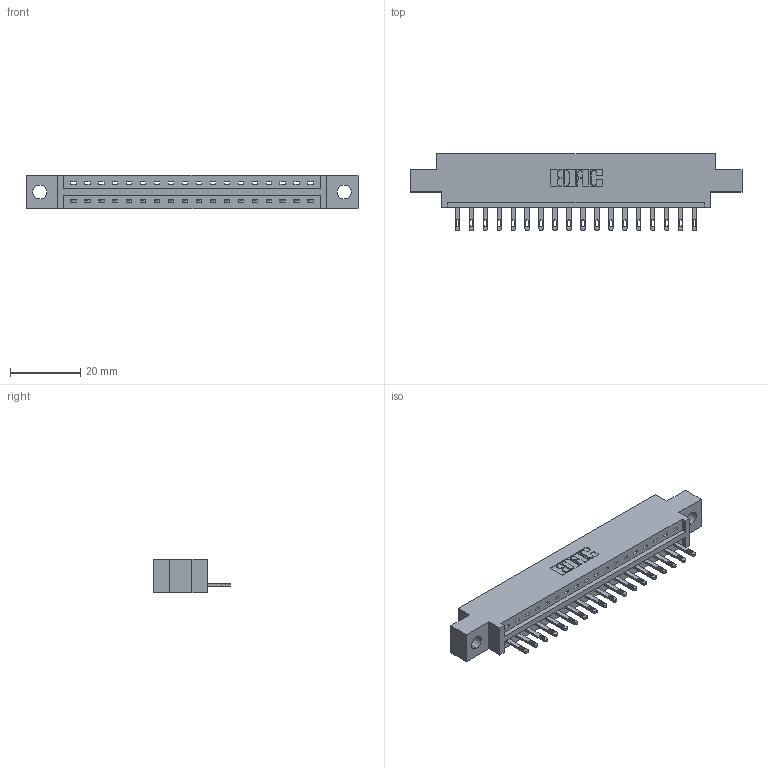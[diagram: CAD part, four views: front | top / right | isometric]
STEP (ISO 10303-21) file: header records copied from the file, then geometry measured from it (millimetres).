
FILE_DESCRIPTION (( 'STEP AP203' ), '1' );
FILE_NAME ('337-018-500-604.STEP', '2019-09-28T19:30:54', ( '' ), ( '' ), 'SwSTEP 2.0', 'SolidWorks 2016', '' );
FILE_SCHEMA (( 'CONFIG_CONTROL_DESIGN' ));
Length unit declared in the file: inch
Products named in the file (3): 337 Part_0.170 Offset - 0.156 Dia-TH; 345-292-001_345-293-100; 337-018-500-604
Assembly tree (19 placements, depth 2):
  337-018-500-604
    337 Part_0.170 Offset - 0.156 Dia-TH
    345-292-001_345-293-100  x18
Bounding box: 94.34 x 21.85 x 9.4 mm (x, y, z)
Volume: 9310 mm3; surface area: 9421.1 mm2
Topology: 19 solids, 19 shells, 1162 faces, 3563 edges, 2374 vertices
Faces by surface type: plane 794, cylinder 368
Entity records: 16549 total; most frequent: CARTESIAN_POINT 2888, ORIENTED_EDGE 2842, DIRECTION 2481, EDGE_CURVE 1421, VECTOR 1289, LINE 1289, VERTEX_POINT 946, AXIS2_PLACEMENT_3D 596
